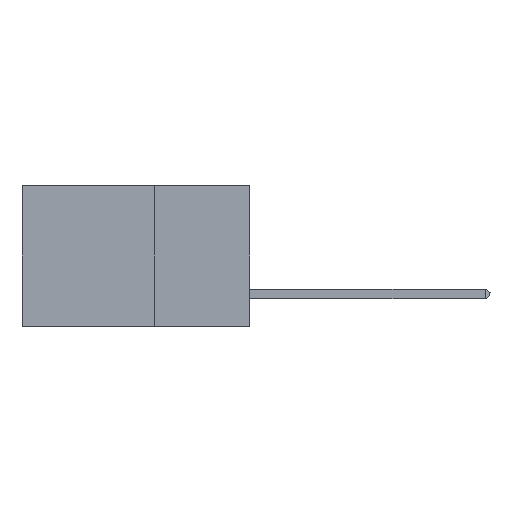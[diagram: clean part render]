
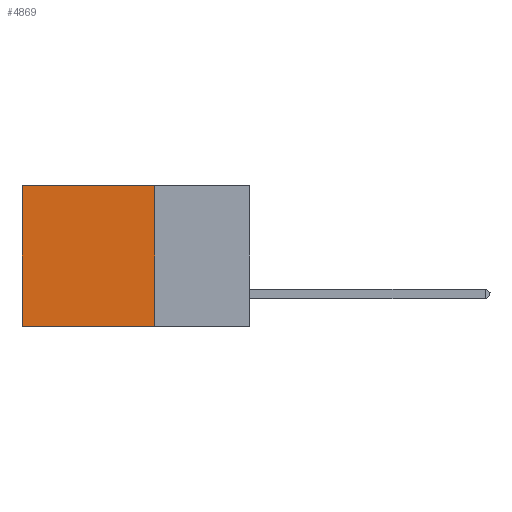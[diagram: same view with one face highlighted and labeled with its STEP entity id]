
A CAD part, left-side view. The second image highlights one B-rep face of the part: STEP entity #4869.
In plain terms, the highlighted planar face has unit normal (-1, 0, 0).
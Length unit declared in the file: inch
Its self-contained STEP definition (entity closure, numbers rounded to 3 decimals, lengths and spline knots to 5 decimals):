
#726 = CARTESIAN_POINT ( 'NONE',  ( 0.2875, 0.25, 0. ) ) ;
#1563 = VERTEX_POINT ( 'NONE', #2242 ) ;
#2003 = DIRECTION ( 'NONE',  ( 0., 0., -1. ) ) ;
#2242 = CARTESIAN_POINT ( 'NONE',  ( 0.2875, 0.6, 0. ) ) ;
#2359 = ORIENTED_EDGE ( 'NONE', *, *, #17363, .T. ) ;
#2404 = CARTESIAN_POINT ( 'NONE',  ( 0.2875, 0.25, 0. ) ) ;
#2448 = CARTESIAN_POINT ( 'NONE',  ( 0.2875, 0.25, -0.37 ) ) ;
#3295 = VECTOR ( 'NONE', #17513, 39.37008 ) ;
#4092 = VECTOR ( 'NONE', #7530, 39.37008 ) ;
#4185 = CARTESIAN_POINT ( 'NONE',  ( 0.2875, 0.25, 0. ) ) ;
#4218 = EDGE_LOOP ( 'NONE', ( #12038, #10182, #20422, #2359 ) ) ;
#4869 = ADVANCED_FACE ( 'NONE', ( #12629 ), #13656, .F. ) ;
#5539 = LINE ( 'NONE', #19131, #4092 ) ;
#5616 = CARTESIAN_POINT ( 'NONE',  ( 0.2875, 0.25, -0.37 ) ) ;
#6687 = VERTEX_POINT ( 'NONE', #19797 ) ;
#7530 = DIRECTION ( 'NONE',  ( 0., 1., 0. ) ) ;
#7754 = VECTOR ( 'NONE', #10320, 39.37008 ) ;
#10182 = ORIENTED_EDGE ( 'NONE', *, *, #25603, .F. ) ;
#10320 = DIRECTION ( 'NONE',  ( 0., 1., 0. ) ) ;
#12038 = ORIENTED_EDGE ( 'NONE', *, *, #14226, .T. ) ;
#12629 = FACE_OUTER_BOUND ( 'NONE', #4218, .T. ) ;
#13656 = PLANE ( 'NONE',  #17747 ) ;
#13983 = LINE ( 'NONE', #2404, #26387 ) ;
#14226 = EDGE_CURVE ( 'NONE', #1563, #6687, #21441, .T. ) ;
#17363 = EDGE_CURVE ( 'NONE', #24483, #1563, #5539, .T. ) ;
#17513 = DIRECTION ( 'NONE',  ( 0., 0., -1. ) ) ;
#17747 = AXIS2_PLACEMENT_3D ( 'NONE', #4185, #25056, #2003 ) ;
#17906 = EDGE_CURVE ( 'NONE', #24483, #21091, #13983, .T. ) ;
#19131 = CARTESIAN_POINT ( 'NONE',  ( 0.2875, 0.25, 0. ) ) ;
#19797 = CARTESIAN_POINT ( 'NONE',  ( 0.2875, 0.6, -0.37 ) ) ;
#20267 = LINE ( 'NONE', #5616, #7754 ) ;
#20422 = ORIENTED_EDGE ( 'NONE', *, *, #17906, .F. ) ;
#21091 = VERTEX_POINT ( 'NONE', #2448 ) ;
#21441 = LINE ( 'NONE', #27895, #3295 ) ;
#23490 = DIRECTION ( 'NONE',  ( 0., 0., -1. ) ) ;
#24483 = VERTEX_POINT ( 'NONE', #726 ) ;
#25056 = DIRECTION ( 'NONE',  ( 1., 0., 0. ) ) ;
#25603 = EDGE_CURVE ( 'NONE', #21091, #6687, #20267, .T. ) ;
#26387 = VECTOR ( 'NONE', #23490, 39.37008 ) ;
#27895 = CARTESIAN_POINT ( 'NONE',  ( 0.2875, 0.6, 0. ) ) ;
